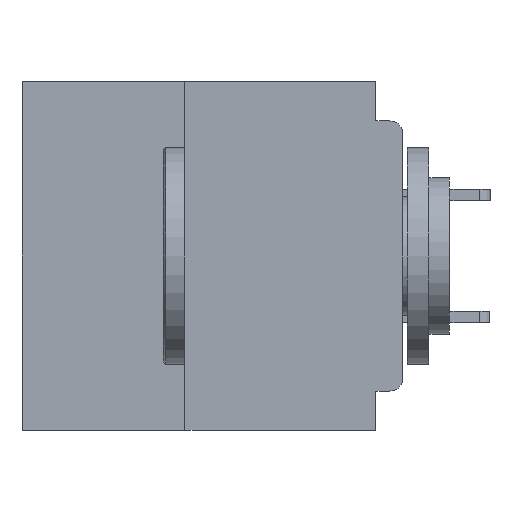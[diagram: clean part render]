
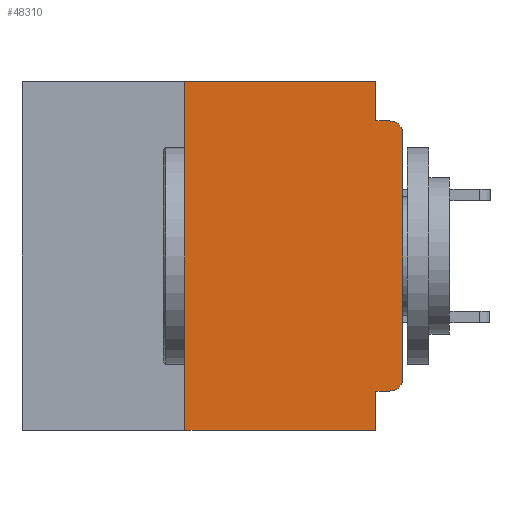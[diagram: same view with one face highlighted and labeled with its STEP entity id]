
A CAD part, left-side view. The second image highlights one B-rep face of the part: STEP entity #48310.
In plain terms, the highlighted planar face has unit normal (-1, 0, 0).
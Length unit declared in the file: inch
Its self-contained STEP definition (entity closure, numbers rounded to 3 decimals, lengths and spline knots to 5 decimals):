
#800 = CARTESIAN_POINT ( 'NONE',  ( 0., 0., -0.34 ) ) ;
#1138 = LINE ( 'NONE', #54819, #22984 ) ;
#1276 = EDGE_CURVE ( 'NONE', #52729, #43684, #24155, .T. ) ;
#2278 = CARTESIAN_POINT ( 'NONE',  ( 0., 0.437, 0. ) ) ;
#2911 = DIRECTION ( 'NONE',  ( 0., 0., 1. ) ) ;
#3514 = CARTESIAN_POINT ( 'NONE',  ( 0., 0., -0.045 ) ) ;
#4082 = CARTESIAN_POINT ( 'NONE',  ( 0., 0., -0.06 ) ) ;
#4672 = ORIENTED_EDGE ( 'NONE', *, *, #19190, .F. ) ;
#7598 = VERTEX_POINT ( 'NONE', #54530 ) ;
#7780 = CARTESIAN_POINT ( 'NONE',  ( 0., 0.031, -0.4 ) ) ;
#7825 = EDGE_CURVE ( 'NONE', #8828, #24653, #32075, .T. ) ;
#7916 = VECTOR ( 'NONE', #25237, 39.37008 ) ;
#7980 = CARTESIAN_POINT ( 'NONE',  ( 0., 0.015, -0.34 ) ) ;
#8319 = CARTESIAN_POINT ( 'NONE',  ( 0., 0.031, -0.4 ) ) ;
#8828 = VERTEX_POINT ( 'NONE', #41593 ) ;
#9248 = EDGE_CURVE ( 'NONE', #48124, #52729, #29726, .T. ) ;
#9636 = EDGE_CURVE ( 'NONE', #16080, #43684, #20915, .T. ) ;
#10773 = EDGE_CURVE ( 'NONE', #8828, #48124, #38215, .T. ) ;
#11096 = ORIENTED_EDGE ( 'NONE', *, *, #10773, .T. ) ;
#12204 = DIRECTION ( 'NONE',  ( 0., 0., -1. ) ) ;
#12408 = DIRECTION ( 'NONE',  ( 0., 0., -1. ) ) ;
#12867 = EDGE_CURVE ( 'NONE', #50048, #16080, #45543, .T. ) ;
#13145 = AXIS2_PLACEMENT_3D ( 'NONE', #19726, #19677, #18970 ) ;
#13688 = CARTESIAN_POINT ( 'NONE',  ( 0., 0.031, 0. ) ) ;
#15186 = VERTEX_POINT ( 'NONE', #8319 ) ;
#15478 = DIRECTION ( 'NONE',  ( 0., -1., 0. ) ) ;
#16080 = VERTEX_POINT ( 'NONE', #31573 ) ;
#17093 = DIRECTION ( 'NONE',  ( 0., 1., 0. ) ) ;
#18028 = EDGE_CURVE ( 'NONE', #7598, #50048, #20418, .T. ) ;
#18096 = DIRECTION ( 'NONE',  ( 0., 0., 1. ) ) ;
#18270 = ORIENTED_EDGE ( 'NONE', *, *, #40301, .T. ) ;
#18970 = DIRECTION ( 'NONE',  ( 0., 0., -1. ) ) ;
#19190 = EDGE_CURVE ( 'NONE', #34403, #7598, #1138, .T. ) ;
#19488 = PLANE ( 'NONE',  #50523 ) ;
#19677 = DIRECTION ( 'NONE',  ( -1., 0., 0. ) ) ;
#19726 = CARTESIAN_POINT ( 'NONE',  ( 0., 0.015, -0.06 ) ) ;
#20418 = LINE ( 'NONE', #2278, #54878 ) ;
#20915 = LINE ( 'NONE', #3514, #7916 ) ;
#21094 = CARTESIAN_POINT ( 'NONE',  ( 0., 0.031, 0. ) ) ;
#22551 = VECTOR ( 'NONE', #34086, 39.37008 ) ;
#22984 = VECTOR ( 'NONE', #2911, 39.37008 ) ;
#23846 = DIRECTION ( 'NONE',  ( 1., 0., 0. ) ) ;
#24115 = FACE_OUTER_BOUND ( 'NONE', #50724, .T. ) ;
#24155 = CIRCLE ( 'NONE', #13145, 0.015 ) ;
#24653 = VERTEX_POINT ( 'NONE', #32490 ) ;
#25237 = DIRECTION ( 'NONE',  ( 0., -1., 0. ) ) ;
#29154 = ORIENTED_EDGE ( 'NONE', *, *, #35708, .F. ) ;
#29384 = LINE ( 'NONE', #53267, #39519 ) ;
#29726 = LINE ( 'NONE', #30956, #39877 ) ;
#30956 = CARTESIAN_POINT ( 'NONE',  ( 0., 0., 0. ) ) ;
#31573 = CARTESIAN_POINT ( 'NONE',  ( 0., 0.031, -0.045 ) ) ;
#32075 = LINE ( 'NONE', #56027, #55052 ) ;
#32490 = CARTESIAN_POINT ( 'NONE',  ( 0., 0.031, -0.355 ) ) ;
#33920 = ORIENTED_EDGE ( 'NONE', *, *, #18028, .F. ) ;
#34086 = DIRECTION ( 'NONE',  ( 0., 0., -1. ) ) ;
#34403 = VERTEX_POINT ( 'NONE', #44924 ) ;
#35192 = ORIENTED_EDGE ( 'NONE', *, *, #12867, .F. ) ;
#35708 = EDGE_CURVE ( 'NONE', #24653, #15186, #37942, .T. ) ;
#37942 = LINE ( 'NONE', #7780, #48108 ) ;
#38215 = CIRCLE ( 'NONE', #40908, 0.015 ) ;
#38319 = DIRECTION ( 'NONE',  ( -1., 0., 0. ) ) ;
#39180 = ORIENTED_EDGE ( 'NONE', *, *, #7825, .F. ) ;
#39519 = VECTOR ( 'NONE', #49125, 39.37008 ) ;
#39877 = VECTOR ( 'NONE', #18096, 39.37008 ) ;
#40301 = EDGE_CURVE ( 'NONE', #34403, #15186, #29384, .T. ) ;
#40908 = AXIS2_PLACEMENT_3D ( 'NONE', #7980, #38319, #12408 ) ;
#41593 = CARTESIAN_POINT ( 'NONE',  ( 0., 0.015, -0.355 ) ) ;
#42393 = ORIENTED_EDGE ( 'NONE', *, *, #9248, .T. ) ;
#43684 = VERTEX_POINT ( 'NONE', #51358 ) ;
#44924 = CARTESIAN_POINT ( 'NONE',  ( 0., 0.25, -0.4 ) ) ;
#45543 = LINE ( 'NONE', #21094, #22551 ) ;
#48108 = VECTOR ( 'NONE', #12204, 39.37008 ) ;
#48124 = VERTEX_POINT ( 'NONE', #800 ) ;
#48310 = ADVANCED_FACE ( 'NONE', ( #24115 ), #19488, .F. ) ;
#49125 = DIRECTION ( 'NONE',  ( 0., -1., 0. ) ) ;
#49738 = CARTESIAN_POINT ( 'NONE',  ( 0., 0.437, 0. ) ) ;
#50048 = VERTEX_POINT ( 'NONE', #13688 ) ;
#50523 = AXIS2_PLACEMENT_3D ( 'NONE', #49738, #23846, #54054 ) ;
#50724 = EDGE_LOOP ( 'NONE', ( #42393, #54404, #51210, #35192, #33920, #4672, #18270, #29154, #39180, #11096 ) ) ;
#51210 = ORIENTED_EDGE ( 'NONE', *, *, #9636, .F. ) ;
#51358 = CARTESIAN_POINT ( 'NONE',  ( 0., 0.015, -0.045 ) ) ;
#52729 = VERTEX_POINT ( 'NONE', #4082 ) ;
#53267 = CARTESIAN_POINT ( 'NONE',  ( 0., 0.437, -0.4 ) ) ;
#54054 = DIRECTION ( 'NONE',  ( 0., 0., -1. ) ) ;
#54404 = ORIENTED_EDGE ( 'NONE', *, *, #1276, .T. ) ;
#54530 = CARTESIAN_POINT ( 'NONE',  ( 0., 0.25, 0. ) ) ;
#54819 = CARTESIAN_POINT ( 'NONE',  ( 0., 0.25, -0.4 ) ) ;
#54878 = VECTOR ( 'NONE', #15478, 39.37008 ) ;
#55052 = VECTOR ( 'NONE', #17093, 39.37008 ) ;
#56027 = CARTESIAN_POINT ( 'NONE',  ( 0., 0., -0.355 ) ) ;
